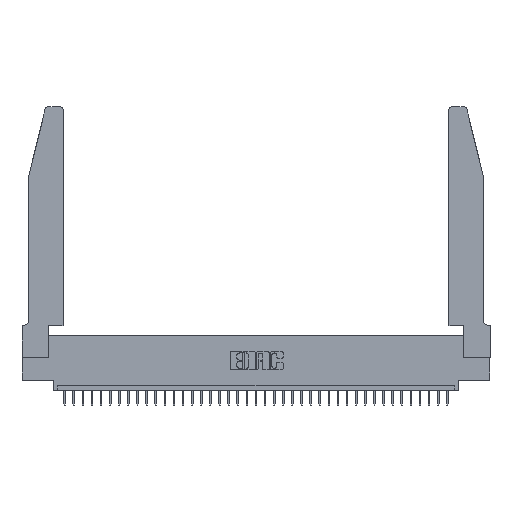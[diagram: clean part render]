
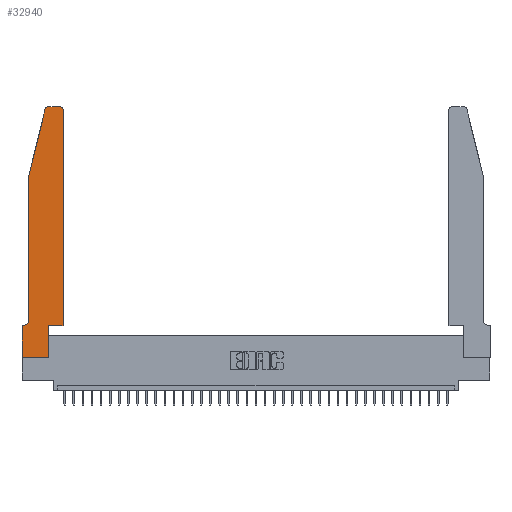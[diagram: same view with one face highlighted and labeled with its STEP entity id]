
A CAD part, top view. The second image highlights one B-rep face of the part: STEP entity #32940.
In plain terms, the highlighted planar face has unit normal (0, 0, 1).
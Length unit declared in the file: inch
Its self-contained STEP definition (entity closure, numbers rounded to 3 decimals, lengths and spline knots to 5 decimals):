
#181 = CIRCLE ( 'NONE', #22478, 0.03 ) ;
#547 = LINE ( 'NONE', #12157, #32922 ) ;
#566 = DIRECTION ( 'NONE',  ( 1., 0., 0. ) ) ;
#1076 = ORIENTED_EDGE ( 'NONE', *, *, #33592, .T. ) ;
#2318 = DIRECTION ( 'NONE',  ( 1., 0., 0. ) ) ;
#2338 = ORIENTED_EDGE ( 'NONE', *, *, #9953, .T. ) ;
#2779 = VECTOR ( 'NONE', #14085, 39.37008 ) ;
#2846 = VERTEX_POINT ( 'NONE', #5373 ) ;
#3217 = ORIENTED_EDGE ( 'NONE', *, *, #5253, .T. ) ;
#3352 = DIRECTION ( 'NONE',  ( 0., 0., 1. ) ) ;
#4084 = CARTESIAN_POINT ( 'NONE',  ( 0.0055, 0.35, 0.37 ) ) ;
#4336 = VERTEX_POINT ( 'NONE', #36807 ) ;
#4546 = CARTESIAN_POINT ( 'NONE',  ( 0.2605, 2.75, 0.37 ) ) ;
#4621 = DIRECTION ( 'NONE',  ( 0., -1., 0. ) ) ;
#4696 = ORIENTED_EDGE ( 'NONE', *, *, #20418, .T. ) ;
#4782 = VECTOR ( 'NONE', #16421, 39.37008 ) ;
#5165 = FACE_OUTER_BOUND ( 'NONE', #16803, .T. ) ;
#5253 = EDGE_CURVE ( 'NONE', #28894, #4336, #36804, .T. ) ;
#5373 = CARTESIAN_POINT ( 'NONE',  ( 0.0755, 2., 0.37 ) ) ;
#5401 = ORIENTED_EDGE ( 'NONE', *, *, #21472, .T. ) ;
#6168 = ORIENTED_EDGE ( 'NONE', *, *, #15358, .T. ) ;
#6278 = CARTESIAN_POINT ( 'NONE',  ( 0.0755, 2., 0.37 ) ) ;
#6802 = VERTEX_POINT ( 'NONE', #15345 ) ;
#7233 = CARTESIAN_POINT ( 'NONE',  ( 0.0755, 0.35, 0.37 ) ) ;
#8096 = ORIENTED_EDGE ( 'NONE', *, *, #32739, .T. ) ;
#9234 = CARTESIAN_POINT ( 'NONE',  ( 0.4205, 2.72, 0.37 ) ) ;
#9591 = ORIENTED_EDGE ( 'NONE', *, *, #14998, .T. ) ;
#9651 = DIRECTION ( 'NONE',  ( -0.239, -0.971, 0. ) ) ;
#9820 = CARTESIAN_POINT ( 'NONE',  ( 0., 0.35, 0.37 ) ) ;
#9953 = EDGE_CURVE ( 'NONE', #29295, #18210, #14140, .T. ) ;
#9985 = CARTESIAN_POINT ( 'NONE',  ( 0.4205, 2.75, 0.37 ) ) ;
#10883 = AXIS2_PLACEMENT_3D ( 'NONE', #12203, #23489, #32252 ) ;
#11750 = LINE ( 'NONE', #15186, #2779 ) ;
#12157 = CARTESIAN_POINT ( 'NONE',  ( 0.0755, 2., 0.37 ) ) ;
#12203 = CARTESIAN_POINT ( 'NONE',  ( 0.0055, 0.42, 0.37 ) ) ;
#12559 = EDGE_CURVE ( 'NONE', #2846, #27191, #16220, .T. ) ;
#12633 = DIRECTION ( 'NONE',  ( -1., 0., 0. ) ) ;
#12693 = LINE ( 'NONE', #36309, #26559 ) ;
#12751 = CARTESIAN_POINT ( 'NONE',  ( 0.0755, 0.42, 0.37 ) ) ;
#13489 = PLANE ( 'NONE',  #19361 ) ;
#13509 = LINE ( 'NONE', #28524, #34083 ) ;
#14041 = VERTEX_POINT ( 'NONE', #35619 ) ;
#14085 = DIRECTION ( 'NONE',  ( 1., 0., 0. ) ) ;
#14140 = LINE ( 'NONE', #7233, #31545 ) ;
#14759 = CARTESIAN_POINT ( 'NONE',  ( 0.25487, 2.72718, 0.37 ) ) ;
#14998 = EDGE_CURVE ( 'NONE', #35351, #6802, #31628, .T. ) ;
#15024 = CIRCLE ( 'NONE', #10883, 0.07 ) ;
#15186 = CARTESIAN_POINT ( 'NONE',  ( 0.4505, 0.35, 0.37 ) ) ;
#15210 = DIRECTION ( 'NONE',  ( 0., -1., 0. ) ) ;
#15345 = CARTESIAN_POINT ( 'NONE',  ( 0.4505, 2.72, 0.37 ) ) ;
#15358 = EDGE_CURVE ( 'NONE', #6802, #21005, #181, .T. ) ;
#15924 = CARTESIAN_POINT ( 'NONE',  ( 0.4505, 0.35, 0.37 ) ) ;
#15930 = VECTOR ( 'NONE', #17501, 39.37008 ) ;
#16033 = CARTESIAN_POINT ( 'NONE',  ( 0., 0.35, 0.37 ) ) ;
#16220 = LINE ( 'NONE', #6278, #34957 ) ;
#16266 = VECTOR ( 'NONE', #22344, 39.37008 ) ;
#16421 = DIRECTION ( 'NONE',  ( 0., 1., 0. ) ) ;
#16803 = EDGE_LOOP ( 'NONE', ( #1076, #4696, #17908, #25461, #8096, #2338, #36983, #5401, #3217, #37116, #9591, #6168 ) ) ;
#16834 = CARTESIAN_POINT ( 'NONE',  ( 0.2865, 0.35, 0.37 ) ) ;
#17185 = CARTESIAN_POINT ( 'NONE',  ( 0.2865, 0., 0.37 ) ) ;
#17501 = DIRECTION ( 'NONE',  ( -1., 0., 0. ) ) ;
#17908 = ORIENTED_EDGE ( 'NONE', *, *, #33362, .T. ) ;
#18210 = VERTEX_POINT ( 'NONE', #9820 ) ;
#19306 = AXIS2_PLACEMENT_3D ( 'NONE', #28720, #25828, #566 ) ;
#19361 = AXIS2_PLACEMENT_3D ( 'NONE', #16033, #21791, #22167 ) ;
#20418 = EDGE_CURVE ( 'NONE', #31438, #30287, #22978, .T. ) ;
#21005 = VERTEX_POINT ( 'NONE', #9985 ) ;
#21472 = EDGE_CURVE ( 'NONE', #14041, #28894, #13509, .T. ) ;
#21791 = DIRECTION ( 'NONE',  ( 0., 0., 1. ) ) ;
#22167 = DIRECTION ( 'NONE',  ( 1., 0., 0. ) ) ;
#22344 = DIRECTION ( 'NONE',  ( 0., 1., 0. ) ) ;
#22478 = AXIS2_PLACEMENT_3D ( 'NONE', #9234, #3352, #23427 ) ;
#22524 = CARTESIAN_POINT ( 'NONE',  ( 0.284, 2.75, 0.37 ) ) ;
#22916 = EDGE_CURVE ( 'NONE', #18210, #14041, #12693, .T. ) ;
#22978 = CIRCLE ( 'NONE', #19306, 0.03 ) ;
#23084 = EDGE_CURVE ( 'NONE', #4336, #35351, #11750, .T. ) ;
#23427 = DIRECTION ( 'NONE',  ( 1., 0., 0. ) ) ;
#23481 = LINE ( 'NONE', #4546, #15930 ) ;
#23489 = DIRECTION ( 'NONE',  ( 0., 0., -1. ) ) ;
#24787 = CARTESIAN_POINT ( 'NONE',  ( 0.4505, 0.35, 0.37 ) ) ;
#25461 = ORIENTED_EDGE ( 'NONE', *, *, #12559, .T. ) ;
#25828 = DIRECTION ( 'NONE',  ( 0., 0., 1. ) ) ;
#26559 = VECTOR ( 'NONE', #4621, 39.37008 ) ;
#27191 = VERTEX_POINT ( 'NONE', #12751 ) ;
#28524 = CARTESIAN_POINT ( 'NONE',  ( 0., 0., 0.37 ) ) ;
#28720 = CARTESIAN_POINT ( 'NONE',  ( 0.284, 2.72, 0.37 ) ) ;
#28894 = VERTEX_POINT ( 'NONE', #17185 ) ;
#29295 = VERTEX_POINT ( 'NONE', #4084 ) ;
#30287 = VERTEX_POINT ( 'NONE', #14759 ) ;
#31438 = VERTEX_POINT ( 'NONE', #22524 ) ;
#31545 = VECTOR ( 'NONE', #12633, 39.37008 ) ;
#31628 = LINE ( 'NONE', #15924, #4782 ) ;
#32252 = DIRECTION ( 'NONE',  ( -1., 0., 0. ) ) ;
#32739 = EDGE_CURVE ( 'NONE', #27191, #29295, #15024, .T. ) ;
#32922 = VECTOR ( 'NONE', #9651, 39.37008 ) ;
#32940 = ADVANCED_FACE ( 'NONE', ( #5165 ), #13489, .T. ) ;
#33362 = EDGE_CURVE ( 'NONE', #30287, #2846, #547, .T. ) ;
#33592 = EDGE_CURVE ( 'NONE', #21005, #31438, #23481, .T. ) ;
#34083 = VECTOR ( 'NONE', #2318, 39.37008 ) ;
#34957 = VECTOR ( 'NONE', #15210, 39.37008 ) ;
#35351 = VERTEX_POINT ( 'NONE', #24787 ) ;
#35619 = CARTESIAN_POINT ( 'NONE',  ( 0., 0., 0.37 ) ) ;
#36309 = CARTESIAN_POINT ( 'NONE',  ( 0., 0., 0.37 ) ) ;
#36804 = LINE ( 'NONE', #16834, #16266 ) ;
#36807 = CARTESIAN_POINT ( 'NONE',  ( 0.2865, 0.35, 0.37 ) ) ;
#36983 = ORIENTED_EDGE ( 'NONE', *, *, #22916, .T. ) ;
#37116 = ORIENTED_EDGE ( 'NONE', *, *, #23084, .T. ) ;
